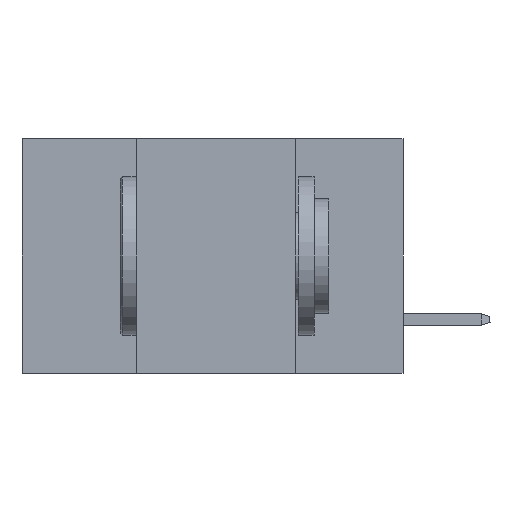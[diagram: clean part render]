
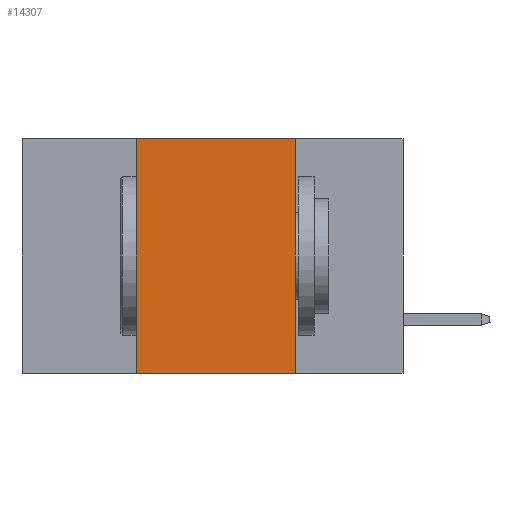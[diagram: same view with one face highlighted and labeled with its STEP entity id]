
A CAD part, left-side view. The second image highlights one B-rep face of the part: STEP entity #14307.
In plain terms, the highlighted planar face has unit normal (-1, 0, 0).
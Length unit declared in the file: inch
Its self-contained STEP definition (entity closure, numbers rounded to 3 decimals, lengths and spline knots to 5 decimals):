
#229 = ORIENTED_EDGE ( 'NONE', *, *, #13836, .F. ) ;
#1094 = LINE ( 'NONE', #4093, #8750 ) ;
#1422 = DIRECTION ( 'NONE',  ( 0., 0., -1. ) ) ;
#1623 = EDGE_LOOP ( 'NONE', ( #28946, #21899, #229, #14559 ) ) ;
#2410 = VERTEX_POINT ( 'NONE', #17059 ) ;
#4093 = CARTESIAN_POINT ( 'NONE',  ( 0., 0.6, 0. ) ) ;
#4164 = AXIS2_PLACEMENT_3D ( 'NONE', #44199, #36361, #1422 ) ;
#5555 = CARTESIAN_POINT ( 'NONE',  ( 0., 0.42, 0. ) ) ;
#6320 = VECTOR ( 'NONE', #36923, 39.37008 ) ;
#8095 = VERTEX_POINT ( 'NONE', #35768 ) ;
#8750 = VECTOR ( 'NONE', #36050, 39.37008 ) ;
#12981 = VERTEX_POINT ( 'NONE', #39987 ) ;
#13567 = EDGE_CURVE ( 'NONE', #2410, #12981, #26367, .T. ) ;
#13802 = CARTESIAN_POINT ( 'NONE',  ( 0., 0.17, 0. ) ) ;
#13836 = EDGE_CURVE ( 'NONE', #2410, #15597, #31826, .T. ) ;
#14307 = ADVANCED_FACE ( 'NONE', ( #32914 ), #30155, .F. ) ;
#14559 = ORIENTED_EDGE ( 'NONE', *, *, #13567, .T. ) ;
#14790 = DIRECTION ( 'NONE',  ( 0., 0., 1. ) ) ;
#15597 = VERTEX_POINT ( 'NONE', #5555 ) ;
#17059 = CARTESIAN_POINT ( 'NONE',  ( 0., 0.42, -0.37 ) ) ;
#19017 = CARTESIAN_POINT ( 'NONE',  ( 0., 0.6, -0.37 ) ) ;
#21899 = ORIENTED_EDGE ( 'NONE', *, *, #24462, .F. ) ;
#24462 = EDGE_CURVE ( 'NONE', #15597, #8095, #1094, .T. ) ;
#25431 = VECTOR ( 'NONE', #14790, 39.37008 ) ;
#26367 = LINE ( 'NONE', #19017, #6320 ) ;
#26749 = VECTOR ( 'NONE', #38213, 39.37008 ) ;
#28452 = EDGE_CURVE ( 'NONE', #8095, #12981, #31302, .T. ) ;
#28946 = ORIENTED_EDGE ( 'NONE', *, *, #28452, .F. ) ;
#30155 = PLANE ( 'NONE',  #4164 ) ;
#31302 = LINE ( 'NONE', #13802, #26749 ) ;
#31826 = LINE ( 'NONE', #32514, #25431 ) ;
#32514 = CARTESIAN_POINT ( 'NONE',  ( 0., 0.42, 0. ) ) ;
#32914 = FACE_OUTER_BOUND ( 'NONE', #1623, .T. ) ;
#35768 = CARTESIAN_POINT ( 'NONE',  ( 0., 0.17, 0. ) ) ;
#36050 = DIRECTION ( 'NONE',  ( 0., -1., 0. ) ) ;
#36361 = DIRECTION ( 'NONE',  ( 1., 0., 0. ) ) ;
#36923 = DIRECTION ( 'NONE',  ( 0., -1., 0. ) ) ;
#38213 = DIRECTION ( 'NONE',  ( 0., 0., -1. ) ) ;
#39987 = CARTESIAN_POINT ( 'NONE',  ( 0., 0.17, -0.37 ) ) ;
#44199 = CARTESIAN_POINT ( 'NONE',  ( 0., 0.6, 0. ) ) ;
